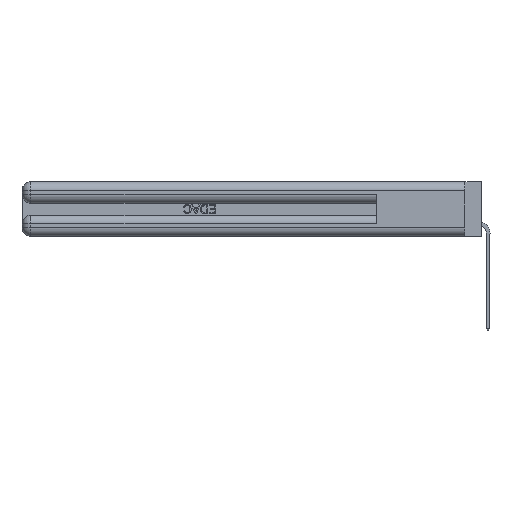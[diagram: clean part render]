
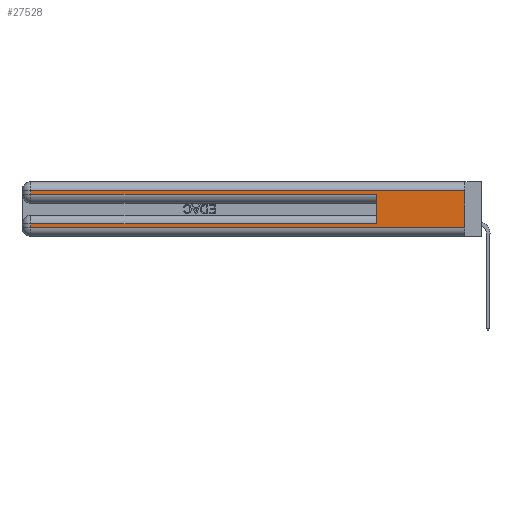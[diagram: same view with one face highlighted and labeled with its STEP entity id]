
A CAD part, left-side view. The second image highlights one B-rep face of the part: STEP entity #27528.
In plain terms, the highlighted planar face has unit normal (-1, 0, 0).
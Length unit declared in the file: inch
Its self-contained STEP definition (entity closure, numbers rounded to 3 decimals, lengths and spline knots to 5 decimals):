
#902 = VECTOR ( 'NONE', #21101, 39.37008 ) ;
#1316 = DIRECTION ( 'NONE',  ( 0., 0., -1. ) ) ;
#2129 = DIRECTION ( 'NONE',  ( 0., 0., -1. ) ) ;
#2614 = EDGE_LOOP ( 'NONE', ( #31800, #27332, #23342, #8686, #22415, #28673, #8335, #19136 ) ) ;
#4305 = CARTESIAN_POINT ( 'NONE',  ( 0., 0., 0.37 ) ) ;
#4569 = CARTESIAN_POINT ( 'NONE',  ( 0., 2.94, 0.31 ) ) ;
#4662 = VECTOR ( 'NONE', #26845, 39.37008 ) ;
#5677 = CARTESIAN_POINT ( 'NONE',  ( 0., 0., 0.285 ) ) ;
#5681 = LINE ( 'NONE', #7277, #27610 ) ;
#5811 = LINE ( 'NONE', #8817, #12483 ) ;
#6270 = VERTEX_POINT ( 'NONE', #26886 ) ;
#6664 = CARTESIAN_POINT ( 'NONE',  ( 0., 2.94, 0.085 ) ) ;
#7277 = CARTESIAN_POINT ( 'NONE',  ( 0., 2.94, 0.37 ) ) ;
#8335 = ORIENTED_EDGE ( 'NONE', *, *, #34942, .T. ) ;
#8686 = ORIENTED_EDGE ( 'NONE', *, *, #10257, .T. ) ;
#8817 = CARTESIAN_POINT ( 'NONE',  ( 0., 0., 0.06 ) ) ;
#9833 = LINE ( 'NONE', #4305, #25480 ) ;
#10257 = EDGE_CURVE ( 'NONE', #25984, #6270, #11380, .T. ) ;
#10521 = VECTOR ( 'NONE', #11641, 39.37008 ) ;
#10780 = EDGE_CURVE ( 'NONE', #17580, #11829, #34538, .T. ) ;
#11000 = VERTEX_POINT ( 'NONE', #27020 ) ;
#11265 = CARTESIAN_POINT ( 'NONE',  ( 0., 0., 0.085 ) ) ;
#11380 = LINE ( 'NONE', #5677, #10521 ) ;
#11641 = DIRECTION ( 'NONE',  ( 0., -1., 0. ) ) ;
#11829 = VERTEX_POINT ( 'NONE', #4569 ) ;
#12201 = LINE ( 'NONE', #26715, #4662 ) ;
#12483 = VECTOR ( 'NONE', #31754, 39.37008 ) ;
#12831 = DIRECTION ( 'NONE',  ( 0., 0., -1. ) ) ;
#12851 = EDGE_CURVE ( 'NONE', #11000, #23247, #13462, .T. ) ;
#13462 = LINE ( 'NONE', #11265, #16585 ) ;
#14445 = VECTOR ( 'NONE', #32677, 39.37008 ) ;
#15440 = CARTESIAN_POINT ( 'NONE',  ( 0., 0., 0.06 ) ) ;
#16116 = EDGE_CURVE ( 'NONE', #11000, #6270, #12201, .T. ) ;
#16585 = VECTOR ( 'NONE', #36921, 39.37008 ) ;
#17224 = FACE_OUTER_BOUND ( 'NONE', #2614, .T. ) ;
#17364 = LINE ( 'NONE', #20855, #902 ) ;
#17580 = VERTEX_POINT ( 'NONE', #23683 ) ;
#17834 = EDGE_CURVE ( 'NONE', #34881, #26815, #5811, .T. ) ;
#18087 = CARTESIAN_POINT ( 'NONE',  ( 0., 0., 0.31 ) ) ;
#19136 = ORIENTED_EDGE ( 'NONE', *, *, #17834, .T. ) ;
#19465 = AXIS2_PLACEMENT_3D ( 'NONE', #36102, #24586, #2129 ) ;
#20855 = CARTESIAN_POINT ( 'NONE',  ( 0., 2.94, 0.37 ) ) ;
#21101 = DIRECTION ( 'NONE',  ( 0., 0., -1. ) ) ;
#22415 = ORIENTED_EDGE ( 'NONE', *, *, #16116, .F. ) ;
#23247 = VERTEX_POINT ( 'NONE', #6664 ) ;
#23342 = ORIENTED_EDGE ( 'NONE', *, *, #33777, .T. ) ;
#23683 = CARTESIAN_POINT ( 'NONE',  ( 0., 0., 0.31 ) ) ;
#24586 = DIRECTION ( 'NONE',  ( 1., 0., 0. ) ) ;
#25480 = VECTOR ( 'NONE', #1316, 39.37008 ) ;
#25984 = VERTEX_POINT ( 'NONE', #36967 ) ;
#26715 = CARTESIAN_POINT ( 'NONE',  ( 0., 0.6, 0.145 ) ) ;
#26815 = VERTEX_POINT ( 'NONE', #15440 ) ;
#26845 = DIRECTION ( 'NONE',  ( 0., 0., 1. ) ) ;
#26886 = CARTESIAN_POINT ( 'NONE',  ( 0., 0.6, 0.285 ) ) ;
#27020 = CARTESIAN_POINT ( 'NONE',  ( 0., 0.6, 0.085 ) ) ;
#27332 = ORIENTED_EDGE ( 'NONE', *, *, #10780, .T. ) ;
#27528 = ADVANCED_FACE ( 'NONE', ( #17224 ), #30333, .F. ) ;
#27610 = VECTOR ( 'NONE', #12831, 39.37008 ) ;
#28673 = ORIENTED_EDGE ( 'NONE', *, *, #12851, .T. ) ;
#29637 = CARTESIAN_POINT ( 'NONE',  ( 0., 2.94, 0.06 ) ) ;
#30333 = PLANE ( 'NONE',  #19465 ) ;
#31754 = DIRECTION ( 'NONE',  ( 0., -1., 0. ) ) ;
#31800 = ORIENTED_EDGE ( 'NONE', *, *, #34885, .F. ) ;
#32677 = DIRECTION ( 'NONE',  ( 0., 1., 0. ) ) ;
#33777 = EDGE_CURVE ( 'NONE', #11829, #25984, #5681, .T. ) ;
#34538 = LINE ( 'NONE', #18087, #14445 ) ;
#34881 = VERTEX_POINT ( 'NONE', #29637 ) ;
#34885 = EDGE_CURVE ( 'NONE', #17580, #26815, #9833, .T. ) ;
#34942 = EDGE_CURVE ( 'NONE', #23247, #34881, #17364, .T. ) ;
#36102 = CARTESIAN_POINT ( 'NONE',  ( 0., 0., 0.37 ) ) ;
#36921 = DIRECTION ( 'NONE',  ( 0., 1., 0. ) ) ;
#36967 = CARTESIAN_POINT ( 'NONE',  ( 0., 2.94, 0.285 ) ) ;
